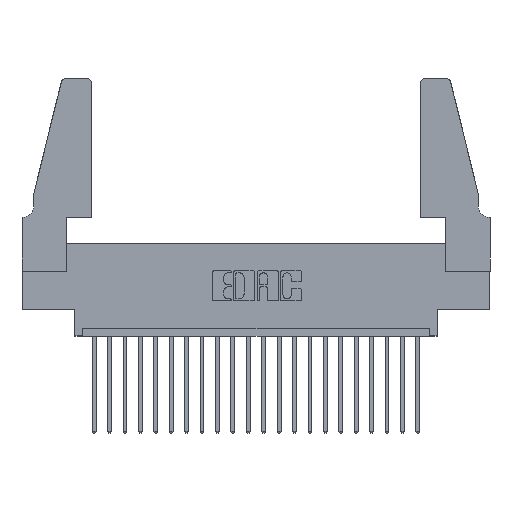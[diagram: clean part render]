
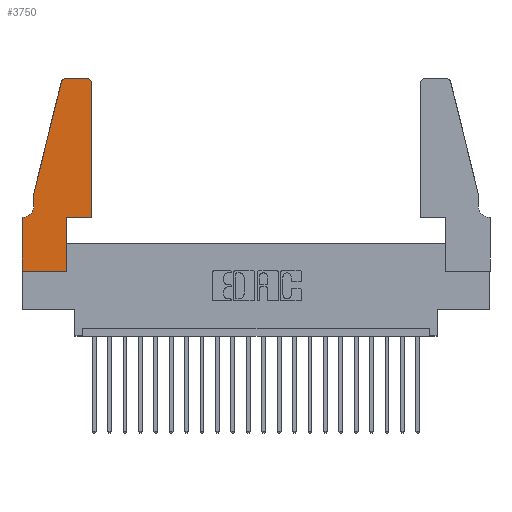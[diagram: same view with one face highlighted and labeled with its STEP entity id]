
A CAD part, top view. The second image highlights one B-rep face of the part: STEP entity #3750.
In plain terms, the highlighted planar face has unit normal (0, 0, 1).
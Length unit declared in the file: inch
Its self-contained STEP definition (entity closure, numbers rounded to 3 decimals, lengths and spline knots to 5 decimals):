
#201 = ORIENTED_EDGE ( 'NONE', *, *, #2105, .T. ) ;
#261 = EDGE_CURVE ( 'NONE', #4507, #5402, #607, .T. ) ;
#304 = DIRECTION ( 'NONE',  ( 0., 1., 0. ) ) ;
#430 = VECTOR ( 'NONE', #12101, 39.37008 ) ;
#515 = DIRECTION ( 'NONE',  ( 1., 0., 0. ) ) ;
#552 = CARTESIAN_POINT ( 'NONE',  ( 0., 0.35, 0.37 ) ) ;
#591 = VECTOR ( 'NONE', #15745, 39.37008 ) ;
#607 = CIRCLE ( 'NONE', #20094, 0.07 ) ;
#971 = LINE ( 'NONE', #11754, #18101 ) ;
#1421 = ORIENTED_EDGE ( 'NONE', *, *, #5971, .T. ) ;
#1605 = DIRECTION ( 'NONE',  ( 0., 0., 1. ) ) ;
#2105 = EDGE_CURVE ( 'NONE', #14009, #15743, #12967, .T. ) ;
#2191 = FACE_OUTER_BOUND ( 'NONE', #2938, .T. ) ;
#2286 = CARTESIAN_POINT ( 'NONE',  ( 0.284, 1.22, 0.37 ) ) ;
#2323 = ORIENTED_EDGE ( 'NONE', *, *, #7433, .T. ) ;
#2468 = VECTOR ( 'NONE', #12248, 39.37008 ) ;
#2495 = DIRECTION ( 'NONE',  ( 1., 0., 0. ) ) ;
#2576 = ORIENTED_EDGE ( 'NONE', *, *, #17430, .T. ) ;
#2938 = EDGE_LOOP ( 'NONE', ( #21358, #16507, #7924, #1421, #20394, #6207, #2323, #15647, #2576, #201, #18741, #13078 ) ) ;
#3041 = CARTESIAN_POINT ( 'NONE',  ( 0.4505, 0.35, 0.37 ) ) ;
#3273 = EDGE_CURVE ( 'NONE', #15743, #12606, #17028, .T. ) ;
#3419 = VERTEX_POINT ( 'NONE', #16089 ) ;
#3499 = AXIS2_PLACEMENT_3D ( 'NONE', #2286, #8923, #18885 ) ;
#3750 = ADVANCED_FACE ( 'NONE', ( #2191 ), #5486, .T. ) ;
#4043 = VERTEX_POINT ( 'NONE', #15014 ) ;
#4078 = CARTESIAN_POINT ( 'NONE',  ( 0.0755, 0.5, 0.37 ) ) ;
#4129 = VECTOR ( 'NONE', #12622, 39.37008 ) ;
#4160 = VECTOR ( 'NONE', #7746, 39.37008 ) ;
#4507 = VERTEX_POINT ( 'NONE', #10892 ) ;
#5123 = CARTESIAN_POINT ( 'NONE',  ( 0.4205, 1.22, 0.37 ) ) ;
#5181 = DIRECTION ( 'NONE',  ( 0., 0., 1. ) ) ;
#5349 = LINE ( 'NONE', #20458, #430 ) ;
#5402 = VERTEX_POINT ( 'NONE', #15211 ) ;
#5486 = PLANE ( 'NONE',  #15114 ) ;
#5641 = VERTEX_POINT ( 'NONE', #4078 ) ;
#5971 = EDGE_CURVE ( 'NONE', #5641, #4507, #15686, .T. ) ;
#6207 = ORIENTED_EDGE ( 'NONE', *, *, #17496, .T. ) ;
#6243 = CARTESIAN_POINT ( 'NONE',  ( 0.4205, 1.25, 0.37 ) ) ;
#6385 = CARTESIAN_POINT ( 'NONE',  ( 0.4505, 1.22, 0.37 ) ) ;
#6889 = CARTESIAN_POINT ( 'NONE',  ( 0.2865, 0.35, 0.37 ) ) ;
#7063 = DIRECTION ( 'NONE',  ( 1., 0., 0. ) ) ;
#7433 = EDGE_CURVE ( 'NONE', #15847, #4043, #10571, .T. ) ;
#7746 = DIRECTION ( 'NONE',  ( 1., 0., 0. ) ) ;
#7924 = ORIENTED_EDGE ( 'NONE', *, *, #8351, .T. ) ;
#8351 = EDGE_CURVE ( 'NONE', #10020, #5641, #9496, .T. ) ;
#8364 = EDGE_CURVE ( 'NONE', #14785, #3419, #5349, .T. ) ;
#8578 = LINE ( 'NONE', #12183, #591 ) ;
#8923 = DIRECTION ( 'NONE',  ( 0., 0., 1. ) ) ;
#9260 = CARTESIAN_POINT ( 'NONE',  ( 0.0055, 0.42, 0.37 ) ) ;
#9368 = VECTOR ( 'NONE', #304, 39.37008 ) ;
#9496 = LINE ( 'NONE', #10482, #10811 ) ;
#10020 = VERTEX_POINT ( 'NONE', #11587 ) ;
#10383 = CARTESIAN_POINT ( 'NONE',  ( 0., 0.35, 0.37 ) ) ;
#10458 = EDGE_CURVE ( 'NONE', #12606, #14785, #18409, .T. ) ;
#10482 = CARTESIAN_POINT ( 'NONE',  ( 0.0755, 0.5, 0.37 ) ) ;
#10571 = LINE ( 'NONE', #19737, #4129 ) ;
#10667 = VECTOR ( 'NONE', #16589, 39.37008 ) ;
#10811 = VECTOR ( 'NONE', #15433, 39.37008 ) ;
#10892 = CARTESIAN_POINT ( 'NONE',  ( 0.0755, 0.42, 0.37 ) ) ;
#11587 = CARTESIAN_POINT ( 'NONE',  ( 0.25487, 1.22718, 0.37 ) ) ;
#11754 = CARTESIAN_POINT ( 'NONE',  ( 0., 0., 0.37 ) ) ;
#12101 = DIRECTION ( 'NONE',  ( -1., 0., 0. ) ) ;
#12183 = CARTESIAN_POINT ( 'NONE',  ( 0.0755, 0.35, 0.37 ) ) ;
#12248 = DIRECTION ( 'NONE',  ( 0., 1., 0. ) ) ;
#12606 = VERTEX_POINT ( 'NONE', #6385 ) ;
#12622 = DIRECTION ( 'NONE',  ( 0., -1., 0. ) ) ;
#12967 = LINE ( 'NONE', #3041, #4160 ) ;
#13078 = ORIENTED_EDGE ( 'NONE', *, *, #10458, .T. ) ;
#14009 = VERTEX_POINT ( 'NONE', #21115 ) ;
#14121 = LINE ( 'NONE', #6889, #9368 ) ;
#14201 = DIRECTION ( 'NONE',  ( 0., 0., -1. ) ) ;
#14785 = VERTEX_POINT ( 'NONE', #6243 ) ;
#15014 = CARTESIAN_POINT ( 'NONE',  ( 0., 0., 0.37 ) ) ;
#15105 = CARTESIAN_POINT ( 'NONE',  ( 0.4505, 0.35, 0.37 ) ) ;
#15114 = AXIS2_PLACEMENT_3D ( 'NONE', #10383, #5181, #7063 ) ;
#15148 = EDGE_CURVE ( 'NONE', #4043, #15795, #971, .T. ) ;
#15211 = CARTESIAN_POINT ( 'NONE',  ( 0.0055, 0.35, 0.37 ) ) ;
#15309 = EDGE_CURVE ( 'NONE', #3419, #10020, #17032, .T. ) ;
#15433 = DIRECTION ( 'NONE',  ( -0.239, -0.971, 0. ) ) ;
#15647 = ORIENTED_EDGE ( 'NONE', *, *, #15148, .T. ) ;
#15686 = LINE ( 'NONE', #20027, #10667 ) ;
#15743 = VERTEX_POINT ( 'NONE', #15105 ) ;
#15745 = DIRECTION ( 'NONE',  ( -1., 0., 0. ) ) ;
#15795 = VERTEX_POINT ( 'NONE', #20570 ) ;
#15847 = VERTEX_POINT ( 'NONE', #552 ) ;
#16089 = CARTESIAN_POINT ( 'NONE',  ( 0.284, 1.25, 0.37 ) ) ;
#16161 = DIRECTION ( 'NONE',  ( -1., 0., 0. ) ) ;
#16507 = ORIENTED_EDGE ( 'NONE', *, *, #15309, .T. ) ;
#16589 = DIRECTION ( 'NONE',  ( 0., -1., 0. ) ) ;
#17028 = LINE ( 'NONE', #18994, #2468 ) ;
#17032 = CIRCLE ( 'NONE', #3499, 0.03 ) ;
#17430 = EDGE_CURVE ( 'NONE', #15795, #14009, #14121, .T. ) ;
#17496 = EDGE_CURVE ( 'NONE', #5402, #15847, #8578, .T. ) ;
#18101 = VECTOR ( 'NONE', #2495, 39.37008 ) ;
#18409 = CIRCLE ( 'NONE', #21193, 0.03 ) ;
#18741 = ORIENTED_EDGE ( 'NONE', *, *, #3273, .T. ) ;
#18885 = DIRECTION ( 'NONE',  ( 1., 0., 0. ) ) ;
#18994 = CARTESIAN_POINT ( 'NONE',  ( 0.4505, 0.35, 0.37 ) ) ;
#19737 = CARTESIAN_POINT ( 'NONE',  ( 0., 0., 0.37 ) ) ;
#20027 = CARTESIAN_POINT ( 'NONE',  ( 0.0755, 0.5, 0.37 ) ) ;
#20094 = AXIS2_PLACEMENT_3D ( 'NONE', #9260, #14201, #16161 ) ;
#20394 = ORIENTED_EDGE ( 'NONE', *, *, #261, .T. ) ;
#20458 = CARTESIAN_POINT ( 'NONE',  ( 0.2605, 1.25, 0.37 ) ) ;
#20570 = CARTESIAN_POINT ( 'NONE',  ( 0.2865, 0., 0.37 ) ) ;
#21115 = CARTESIAN_POINT ( 'NONE',  ( 0.2865, 0.35, 0.37 ) ) ;
#21193 = AXIS2_PLACEMENT_3D ( 'NONE', #5123, #1605, #515 ) ;
#21358 = ORIENTED_EDGE ( 'NONE', *, *, #8364, .T. ) ;
